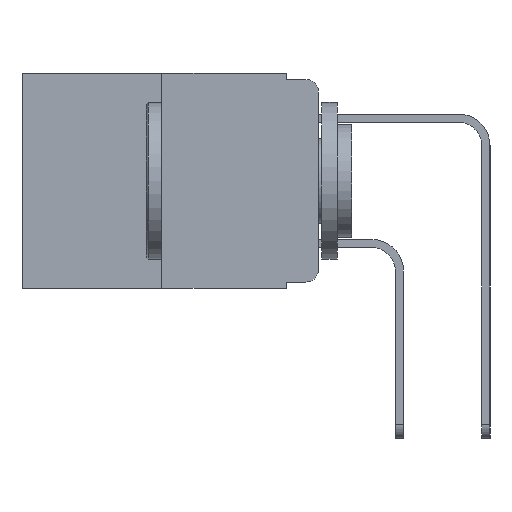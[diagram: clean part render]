
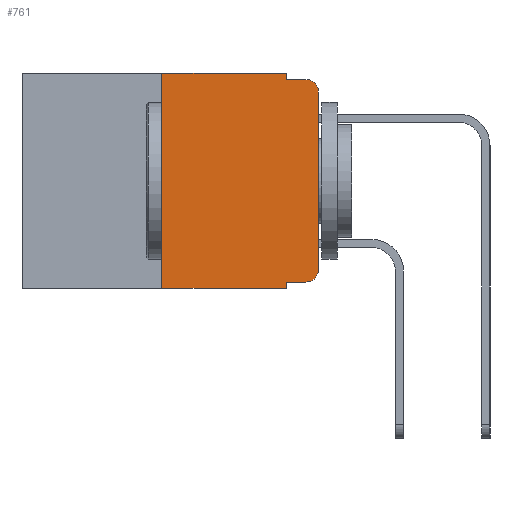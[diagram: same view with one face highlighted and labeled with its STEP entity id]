
A CAD part, left-side view. The second image highlights one B-rep face of the part: STEP entity #761.
In plain terms, the highlighted planar face has unit normal (-1, 0, 0).
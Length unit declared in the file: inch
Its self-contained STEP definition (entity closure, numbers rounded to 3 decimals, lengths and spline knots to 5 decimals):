
#99 = VERTEX_POINT ( 'NONE', #10077 ) ;
#192 = DIRECTION ( 'NONE',  ( -1., 0., 0. ) ) ;
#761 = ADVANCED_FACE ( 'NONE', ( #10109 ), #5846, .F. ) ;
#803 = DIRECTION ( 'NONE',  ( 0., 0., 1. ) ) ;
#841 = ORIENTED_EDGE ( 'NONE', *, *, #7122, .T. ) ;
#1389 = CARTESIAN_POINT ( 'NONE',  ( 0., 0.473, 0. ) ) ;
#1493 = LINE ( 'NONE', #15052, #5163 ) ;
#1644 = LINE ( 'NONE', #4358, #12003 ) ;
#2531 = CARTESIAN_POINT ( 'NONE',  ( 0., 0., -0.313 ) ) ;
#2669 = ORIENTED_EDGE ( 'NONE', *, *, #6240, .T. ) ;
#2909 = VERTEX_POINT ( 'NONE', #3117 ) ;
#3117 = CARTESIAN_POINT ( 'NONE',  ( 0., 0., -0.03 ) ) ;
#3212 = ORIENTED_EDGE ( 'NONE', *, *, #15902, .T. ) ;
#3273 = ORIENTED_EDGE ( 'NONE', *, *, #15057, .T. ) ;
#3303 = VERTEX_POINT ( 'NONE', #9026 ) ;
#3317 = DIRECTION ( 'NONE',  ( -1., 0., 0. ) ) ;
#3511 = CARTESIAN_POINT ( 'NONE',  ( 0., 0.051, 0. ) ) ;
#4358 = CARTESIAN_POINT ( 'NONE',  ( 0., 0.25, 0. ) ) ;
#4703 = DIRECTION ( 'NONE',  ( 0., -1., 0. ) ) ;
#4798 = VERTEX_POINT ( 'NONE', #13379 ) ;
#4894 = DIRECTION ( 'NONE',  ( 0., 0., -1. ) ) ;
#5105 = LINE ( 'NONE', #3511, #11803 ) ;
#5163 = VECTOR ( 'NONE', #5840, 39.37008 ) ;
#5263 = LINE ( 'NONE', #7354, #15357 ) ;
#5479 = LINE ( 'NONE', #12231, #12156 ) ;
#5562 = EDGE_CURVE ( 'NONE', #4798, #3303, #15124, .T. ) ;
#5587 = DIRECTION ( 'NONE',  ( 0., -1., 0. ) ) ;
#5642 = DIRECTION ( 'NONE',  ( 0., -1., 0. ) ) ;
#5645 = ORIENTED_EDGE ( 'NONE', *, *, #8014, .F. ) ;
#5751 = DIRECTION ( 'NONE',  ( 0., 0., 1. ) ) ;
#5840 = DIRECTION ( 'NONE',  ( 0., -1., 0. ) ) ;
#5846 = PLANE ( 'NONE',  #10879 ) ;
#5923 = ORIENTED_EDGE ( 'NONE', *, *, #10708, .F. ) ;
#6147 = DIRECTION ( 'NONE',  ( 1., 0., 0. ) ) ;
#6218 = CARTESIAN_POINT ( 'NONE',  ( 0., 0.02, -0.01 ) ) ;
#6240 = EDGE_CURVE ( 'NONE', #14094, #9307, #11890, .T. ) ;
#6595 = ORIENTED_EDGE ( 'NONE', *, *, #14189, .F. ) ;
#6701 = VERTEX_POINT ( 'NONE', #6218 ) ;
#6807 = CARTESIAN_POINT ( 'NONE',  ( 0., 0.051, 0. ) ) ;
#6969 = AXIS2_PLACEMENT_3D ( 'NONE', #11405, #3317, #12702 ) ;
#7122 = EDGE_CURVE ( 'NONE', #16979, #14094, #1493, .T. ) ;
#7354 = CARTESIAN_POINT ( 'NONE',  ( 0., 0.473, 0. ) ) ;
#8014 = EDGE_CURVE ( 'NONE', #16979, #3303, #5105, .T. ) ;
#8268 = CARTESIAN_POINT ( 'NONE',  ( 0., 0.473, -0.343 ) ) ;
#8358 = CARTESIAN_POINT ( 'NONE',  ( 0., 0.02, -0.313 ) ) ;
#8913 = EDGE_CURVE ( 'NONE', #4798, #11716, #1644, .T. ) ;
#9026 = CARTESIAN_POINT ( 'NONE',  ( 0., 0.051, -0.343 ) ) ;
#9075 = DIRECTION ( 'NONE',  ( 0., 0., -1. ) ) ;
#9307 = VERTEX_POINT ( 'NONE', #2531 ) ;
#9310 = DIRECTION ( 'NONE',  ( 0., 0., -1. ) ) ;
#9720 = DIRECTION ( 'NONE',  ( 0., 0., -1. ) ) ;
#9913 = ORIENTED_EDGE ( 'NONE', *, *, #12053, .F. ) ;
#10077 = CARTESIAN_POINT ( 'NONE',  ( 0., 0.051, 0. ) ) ;
#10109 = FACE_OUTER_BOUND ( 'NONE', #15194, .T. ) ;
#10239 = CARTESIAN_POINT ( 'NONE',  ( 0., 0., 0. ) ) ;
#10708 = EDGE_CURVE ( 'NONE', #99, #14353, #15345, .T. ) ;
#10792 = CARTESIAN_POINT ( 'NONE',  ( 0., 0.02, -0.333 ) ) ;
#10879 = AXIS2_PLACEMENT_3D ( 'NONE', #1389, #6147, #9075 ) ;
#11405 = CARTESIAN_POINT ( 'NONE',  ( 0., 0.02, -0.03 ) ) ;
#11707 = ORIENTED_EDGE ( 'NONE', *, *, #8913, .F. ) ;
#11715 = VECTOR ( 'NONE', #5642, 39.37008 ) ;
#11716 = VERTEX_POINT ( 'NONE', #14635 ) ;
#11722 = CIRCLE ( 'NONE', #6969, 0.02 ) ;
#11803 = VECTOR ( 'NONE', #4894, 39.37008 ) ;
#11890 = CIRCLE ( 'NONE', #16824, 0.02 ) ;
#12003 = VECTOR ( 'NONE', #5751, 39.37008 ) ;
#12053 = EDGE_CURVE ( 'NONE', #11716, #99, #5263, .T. ) ;
#12093 = LINE ( 'NONE', #10239, #15105 ) ;
#12156 = VECTOR ( 'NONE', #5587, 39.37008 ) ;
#12231 = CARTESIAN_POINT ( 'NONE',  ( 0., 0.051, -0.01 ) ) ;
#12702 = DIRECTION ( 'NONE',  ( 0., 0., -1. ) ) ;
#13379 = CARTESIAN_POINT ( 'NONE',  ( 0., 0.25, -0.343 ) ) ;
#13907 = CARTESIAN_POINT ( 'NONE',  ( 0., 0.051, -0.01 ) ) ;
#14094 = VERTEX_POINT ( 'NONE', #10792 ) ;
#14133 = CARTESIAN_POINT ( 'NONE',  ( 0., 0.051, -0.333 ) ) ;
#14165 = ORIENTED_EDGE ( 'NONE', *, *, #5562, .T. ) ;
#14189 = EDGE_CURVE ( 'NONE', #14353, #6701, #5479, .T. ) ;
#14353 = VERTEX_POINT ( 'NONE', #13907 ) ;
#14635 = CARTESIAN_POINT ( 'NONE',  ( 0., 0.25, 0. ) ) ;
#15052 = CARTESIAN_POINT ( 'NONE',  ( 0., 0.051, -0.333 ) ) ;
#15057 = EDGE_CURVE ( 'NONE', #2909, #6701, #11722, .T. ) ;
#15105 = VECTOR ( 'NONE', #803, 39.37008 ) ;
#15124 = LINE ( 'NONE', #8268, #11715 ) ;
#15194 = EDGE_LOOP ( 'NONE', ( #3212, #3273, #6595, #5923, #9913, #11707, #14165, #5645, #841, #2669 ) ) ;
#15345 = LINE ( 'NONE', #6807, #16146 ) ;
#15357 = VECTOR ( 'NONE', #4703, 39.37008 ) ;
#15902 = EDGE_CURVE ( 'NONE', #9307, #2909, #12093, .T. ) ;
#16146 = VECTOR ( 'NONE', #9310, 39.37008 ) ;
#16824 = AXIS2_PLACEMENT_3D ( 'NONE', #8358, #192, #9720 ) ;
#16979 = VERTEX_POINT ( 'NONE', #14133 ) ;
